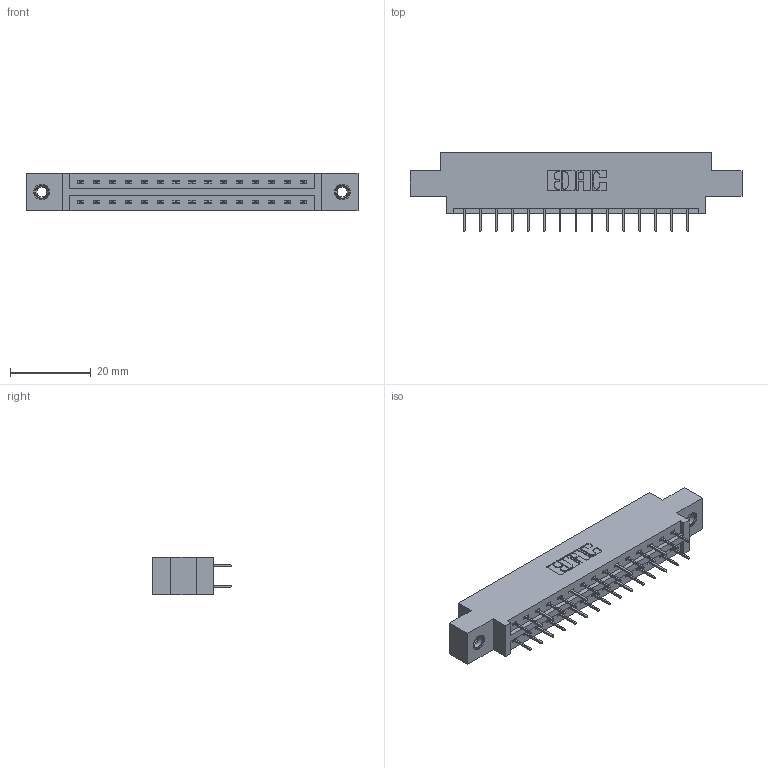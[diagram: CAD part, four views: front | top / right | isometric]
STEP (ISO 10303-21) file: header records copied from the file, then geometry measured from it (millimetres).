
FILE_DESCRIPTION (( 'STEP AP203' ), '1' );
FILE_NAME ('387-030-524-807.STEP', '2019-10-17T14:22:23', ( '' ), ( '' ), 'SwSTEP 2.0', 'SolidWorks 2016', '' );
FILE_SCHEMA (( 'CONFIG_CONTROL_DESIGN' ));
Length unit declared in the file: inch
Products named in the file (4): 337 Part_0.170 Offset - 0.156 Dia-TI; 387-030-524-807; 345-292-001_345-293-124; 345-250-001_345-250-005-103
Assembly tree (33 placements, depth 2):
  387-030-524-807
    337 Part_0.170 Offset - 0.156 Dia-TI
    345-292-001_345-293-124  x30
    345-250-001_345-250-005-103  x2
Bounding box: 82.45 x 19.69 x 9.4 mm (x, y, z)
Volume: 8153.2 mm3; surface area: 8958.2 mm2
Topology: 33 solids, 33 shells, 1918 faces, 5409 edges, 3478 vertices
Faces by surface type: plane 1426, cylinder 476, cone 12, torus 4
Entity records: 16514 total; most frequent: CARTESIAN_POINT 2785, ORIENTED_EDGE 2714, DIRECTION 2451, EDGE_CURVE 1357, VECTOR 1213, LINE 1213, VERTEX_POINT 896, AXIS2_PLACEMENT_3D 619
